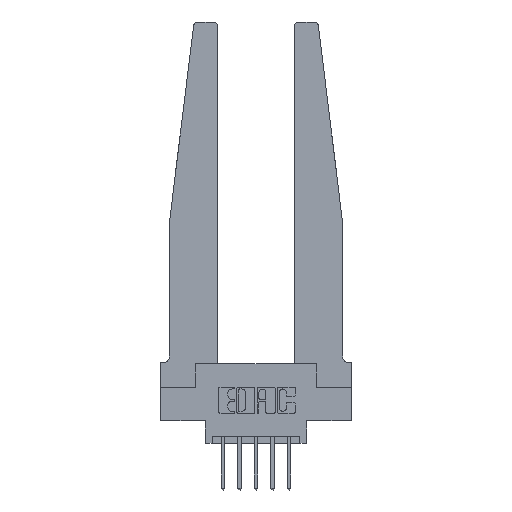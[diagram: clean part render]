
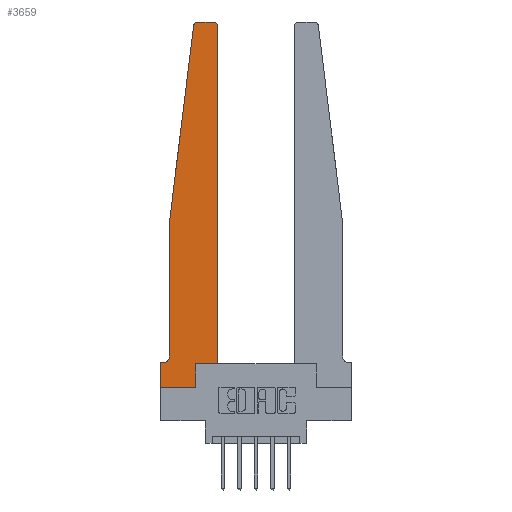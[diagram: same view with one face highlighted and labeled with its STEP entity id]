
A CAD part, top view. The second image highlights one B-rep face of the part: STEP entity #3659.
In plain terms, the highlighted planar face has unit normal (0, 0, 1).
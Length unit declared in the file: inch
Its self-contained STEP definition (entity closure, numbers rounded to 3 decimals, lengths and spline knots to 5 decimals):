
#55 = CARTESIAN_POINT ( 'NONE',  ( 0.395, 2.75, 0.37 ) ) ;
#294 = EDGE_CURVE ( 'NONE', #6415, #1399, #11748, .T. ) ;
#424 = LINE ( 'NONE', #13136, #3624 ) ;
#489 = DIRECTION ( 'NONE',  ( 0., -1., 0. ) ) ;
#549 = CARTESIAN_POINT ( 'NONE',  ( 0.065, 1.25, 0.37 ) ) ;
#797 = EDGE_CURVE ( 'NONE', #6243, #5351, #4887, .T. ) ;
#867 = DIRECTION ( 'NONE',  ( 0., 0., 1. ) ) ;
#925 = VECTOR ( 'NONE', #10860, 39.37008 ) ;
#992 = EDGE_LOOP ( 'NONE', ( #9630, #12088, #3497, #12338, #5265, #9238, #12657, #9587, #2511, #7371, #13320, #10761 ) ) ;
#1028 = CARTESIAN_POINT ( 'NONE',  ( 0.065, 1.25, 0.37 ) ) ;
#1220 = CIRCLE ( 'NONE', #13276, 0.03 ) ;
#1399 = VERTEX_POINT ( 'NONE', #8482 ) ;
#1507 = DIRECTION ( 'NONE',  ( 0., 1., 0. ) ) ;
#1592 = DIRECTION ( 'NONE',  ( -1., 0., 0. ) ) ;
#1899 = CARTESIAN_POINT ( 'NONE',  ( 0.395, 2.72, 0.37 ) ) ;
#2102 = VERTEX_POINT ( 'NONE', #6801 ) ;
#2454 = VECTOR ( 'NONE', #6139, 39.37008 ) ;
#2469 = CARTESIAN_POINT ( 'NONE',  ( 0.425, 0.18, 0.37 ) ) ;
#2511 = ORIENTED_EDGE ( 'NONE', *, *, #13206, .T. ) ;
#2534 = CARTESIAN_POINT ( 'NONE',  ( 0.2605, 0., 0.37 ) ) ;
#2572 = EDGE_CURVE ( 'NONE', #12296, #13535, #8731, .T. ) ;
#2826 = EDGE_CURVE ( 'NONE', #9458, #4133, #8156, .T. ) ;
#3172 = EDGE_CURVE ( 'NONE', #9674, #11226, #12323, .T. ) ;
#3253 = PLANE ( 'NONE',  #12409 ) ;
#3350 = CARTESIAN_POINT ( 'NONE',  ( 0.065, 0.2375, 0.37 ) ) ;
#3497 = ORIENTED_EDGE ( 'NONE', *, *, #2572, .T. ) ;
#3622 = VECTOR ( 'NONE', #1507, 39.37008 ) ;
#3624 = VECTOR ( 'NONE', #1592, 39.37008 ) ;
#3659 = ADVANCED_FACE ( 'NONE', ( #12655 ), #3253, .T. ) ;
#3696 = CARTESIAN_POINT ( 'NONE',  ( 0., 0., 0.37 ) ) ;
#3775 = DIRECTION ( 'NONE',  ( -1., 0., 0. ) ) ;
#4133 = VERTEX_POINT ( 'NONE', #2534 ) ;
#4172 = EDGE_CURVE ( 'NONE', #13535, #4553, #5951, .T. ) ;
#4215 = VECTOR ( 'NONE', #489, 39.37008 ) ;
#4281 = VECTOR ( 'NONE', #4798, 39.37008 ) ;
#4553 = VERTEX_POINT ( 'NONE', #3350 ) ;
#4598 = CARTESIAN_POINT ( 'NONE',  ( 0.2605, 0.18, 0.37 ) ) ;
#4798 = DIRECTION ( 'NONE',  ( -0.122, -0.992, 0. ) ) ;
#4854 = CARTESIAN_POINT ( 'NONE',  ( 0.065, 1.25, 0.37 ) ) ;
#4887 = CIRCLE ( 'NONE', #6637, 0.03 ) ;
#5112 = CARTESIAN_POINT ( 'NONE',  ( 0.015, 0.1875, 0.37 ) ) ;
#5265 = ORIENTED_EDGE ( 'NONE', *, *, #11188, .T. ) ;
#5351 = VERTEX_POINT ( 'NONE', #55 ) ;
#5603 = VECTOR ( 'NONE', #8121, 39.37008 ) ;
#5677 = DIRECTION ( 'NONE',  ( 1., 0., 0. ) ) ;
#5799 = AXIS2_PLACEMENT_3D ( 'NONE', #13117, #10030, #3775 ) ;
#5951 = LINE ( 'NONE', #4854, #8063 ) ;
#6102 = CARTESIAN_POINT ( 'NONE',  ( 0.24675, 2.72367, 0.37 ) ) ;
#6139 = DIRECTION ( 'NONE',  ( -1., 0., 0. ) ) ;
#6243 = VERTEX_POINT ( 'NONE', #11990 ) ;
#6401 = DIRECTION ( 'NONE',  ( 0., 0., 1. ) ) ;
#6415 = VERTEX_POINT ( 'NONE', #5112 ) ;
#6467 = DIRECTION ( 'NONE',  ( 1., 0., 0. ) ) ;
#6637 = AXIS2_PLACEMENT_3D ( 'NONE', #1899, #867, #8007 ) ;
#6680 = LINE ( 'NONE', #10877, #4215 ) ;
#6801 = CARTESIAN_POINT ( 'NONE',  ( 0.27653, 2.75, 0.37 ) ) ;
#7296 = CARTESIAN_POINT ( 'NONE',  ( 0.425, 0.18, 0.37 ) ) ;
#7371 = ORIENTED_EDGE ( 'NONE', *, *, #3172, .T. ) ;
#7416 = CARTESIAN_POINT ( 'NONE',  ( 0., 0.1875, 0.37 ) ) ;
#7550 = CARTESIAN_POINT ( 'NONE',  ( 0.065, 0.1875, 0.37 ) ) ;
#8007 = DIRECTION ( 'NONE',  ( 1., 0., 0. ) ) ;
#8063 = VECTOR ( 'NONE', #10289, 39.37008 ) ;
#8088 = DIRECTION ( 'NONE',  ( 1., 0., 0. ) ) ;
#8121 = DIRECTION ( 'NONE',  ( 1., 0., 0. ) ) ;
#8156 = LINE ( 'NONE', #9141, #12163 ) ;
#8209 = CIRCLE ( 'NONE', #5799, 0.05 ) ;
#8454 = EDGE_CURVE ( 'NONE', #1399, #9458, #6680, .T. ) ;
#8482 = CARTESIAN_POINT ( 'NONE',  ( 0., 0.1875, 0.37 ) ) ;
#8729 = LINE ( 'NONE', #2469, #925 ) ;
#8731 = LINE ( 'NONE', #549, #4281 ) ;
#8868 = EDGE_CURVE ( 'NONE', #11226, #6243, #8729, .T. ) ;
#9141 = CARTESIAN_POINT ( 'NONE',  ( 0., 0., 0.37 ) ) ;
#9238 = ORIENTED_EDGE ( 'NONE', *, *, #294, .T. ) ;
#9458 = VERTEX_POINT ( 'NONE', #3696 ) ;
#9587 = ORIENTED_EDGE ( 'NONE', *, *, #2826, .T. ) ;
#9630 = ORIENTED_EDGE ( 'NONE', *, *, #11838, .T. ) ;
#9674 = VERTEX_POINT ( 'NONE', #10625 ) ;
#9876 = CARTESIAN_POINT ( 'NONE',  ( 0.27653, 2.72, 0.37 ) ) ;
#10030 = DIRECTION ( 'NONE',  ( 0., 0., -1. ) ) ;
#10289 = DIRECTION ( 'NONE',  ( 0., -1., 0. ) ) ;
#10625 = CARTESIAN_POINT ( 'NONE',  ( 0.2605, 0.18, 0.37 ) ) ;
#10761 = ORIENTED_EDGE ( 'NONE', *, *, #797, .T. ) ;
#10860 = DIRECTION ( 'NONE',  ( 0., 1., 0. ) ) ;
#10877 = CARTESIAN_POINT ( 'NONE',  ( 0., 0., 0.37 ) ) ;
#11188 = EDGE_CURVE ( 'NONE', #4553, #6415, #8209, .T. ) ;
#11226 = VERTEX_POINT ( 'NONE', #12611 ) ;
#11748 = LINE ( 'NONE', #7550, #2454 ) ;
#11810 = LINE ( 'NONE', #4598, #3622 ) ;
#11838 = EDGE_CURVE ( 'NONE', #5351, #2102, #424, .T. ) ;
#11990 = CARTESIAN_POINT ( 'NONE',  ( 0.425, 2.72, 0.37 ) ) ;
#12088 = ORIENTED_EDGE ( 'NONE', *, *, #12425, .T. ) ;
#12163 = VECTOR ( 'NONE', #8088, 39.37008 ) ;
#12296 = VERTEX_POINT ( 'NONE', #6102 ) ;
#12323 = LINE ( 'NONE', #7296, #5603 ) ;
#12338 = ORIENTED_EDGE ( 'NONE', *, *, #4172, .T. ) ;
#12409 = AXIS2_PLACEMENT_3D ( 'NONE', #7416, #6401, #6467 ) ;
#12425 = EDGE_CURVE ( 'NONE', #2102, #12296, #1220, .T. ) ;
#12611 = CARTESIAN_POINT ( 'NONE',  ( 0.425, 0.18, 0.37 ) ) ;
#12655 = FACE_OUTER_BOUND ( 'NONE', #992, .T. ) ;
#12657 = ORIENTED_EDGE ( 'NONE', *, *, #8454, .T. ) ;
#12758 = DIRECTION ( 'NONE',  ( 0., 0., 1. ) ) ;
#13117 = CARTESIAN_POINT ( 'NONE',  ( 0.015, 0.2375, 0.37 ) ) ;
#13136 = CARTESIAN_POINT ( 'NONE',  ( 0.25, 2.75, 0.37 ) ) ;
#13206 = EDGE_CURVE ( 'NONE', #4133, #9674, #11810, .T. ) ;
#13276 = AXIS2_PLACEMENT_3D ( 'NONE', #9876, #12758, #5677 ) ;
#13320 = ORIENTED_EDGE ( 'NONE', *, *, #8868, .T. ) ;
#13535 = VERTEX_POINT ( 'NONE', #1028 ) ;
